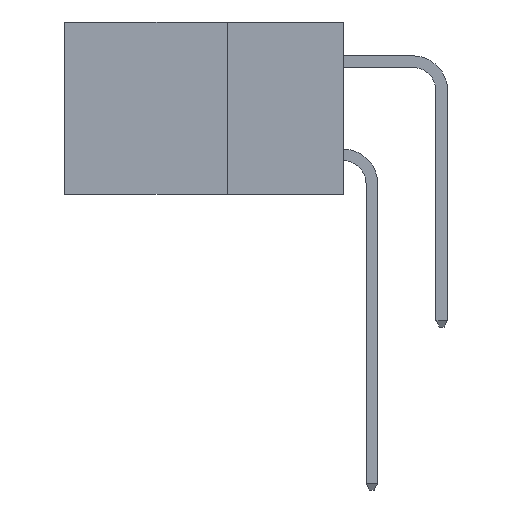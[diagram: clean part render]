
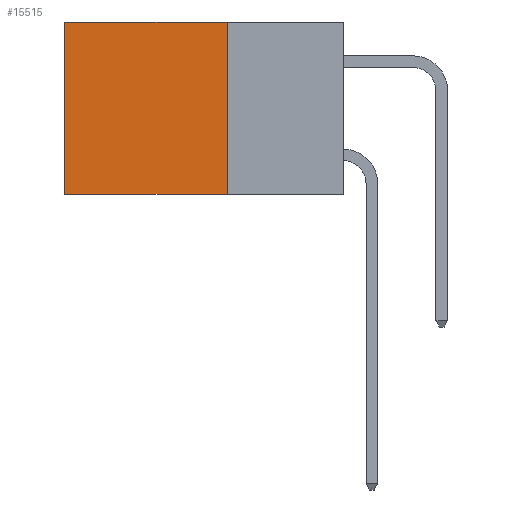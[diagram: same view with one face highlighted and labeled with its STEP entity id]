
A CAD part, left-side view. The second image highlights one B-rep face of the part: STEP entity #15515.
In plain terms, the highlighted planar face has unit normal (-1, 0, 0).
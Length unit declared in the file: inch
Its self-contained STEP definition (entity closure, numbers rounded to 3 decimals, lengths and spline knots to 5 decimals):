
#250 = ORIENTED_EDGE ( 'NONE', *, *, #4271, .F. ) ;
#1023 = FACE_OUTER_BOUND ( 'NONE', #12965, .T. ) ;
#1714 = LINE ( 'NONE', #11186, #11047 ) ;
#1760 = CARTESIAN_POINT ( 'NONE',  ( 0.2615, 0.25, -0.37 ) ) ;
#1818 = DIRECTION ( 'NONE',  ( 0., 1., 0. ) ) ;
#1838 = CARTESIAN_POINT ( 'NONE',  ( 0.2615, 0.25, -0.37 ) ) ;
#2132 = DIRECTION ( 'NONE',  ( 0., 0., -1. ) ) ;
#2157 = CARTESIAN_POINT ( 'NONE',  ( 0.2615, 0.25, 0. ) ) ;
#2179 = DIRECTION ( 'NONE',  ( 1., 0., 0. ) ) ;
#2258 = DIRECTION ( 'NONE',  ( 0., 1., 0. ) ) ;
#2661 = DIRECTION ( 'NONE',  ( 0., 0., -1. ) ) ;
#4271 = EDGE_CURVE ( 'NONE', #15142, #9403, #8372, .T. ) ;
#4823 = VECTOR ( 'NONE', #2258, 39.37008 ) ;
#4864 = CARTESIAN_POINT ( 'NONE',  ( 0.2615, 0.6, -0.37 ) ) ;
#5030 = EDGE_CURVE ( 'NONE', #6784, #15142, #6230, .T. ) ;
#6190 = CARTESIAN_POINT ( 'NONE',  ( 0.2615, 0.25, -0.37 ) ) ;
#6230 = LINE ( 'NONE', #1760, #12434 ) ;
#6784 = VERTEX_POINT ( 'NONE', #9208 ) ;
#8066 = ORIENTED_EDGE ( 'NONE', *, *, #14454, .T. ) ;
#8120 = PLANE ( 'NONE',  #15577 ) ;
#8123 = ORIENTED_EDGE ( 'NONE', *, *, #5030, .F. ) ;
#8372 = LINE ( 'NONE', #1838, #13414 ) ;
#9208 = CARTESIAN_POINT ( 'NONE',  ( 0.2615, 0.25, 0. ) ) ;
#9403 = VERTEX_POINT ( 'NONE', #4864 ) ;
#9445 = CARTESIAN_POINT ( 'NONE',  ( 0.2615, 0.25, -0.37 ) ) ;
#10680 = DIRECTION ( 'NONE',  ( 0., 0., -1. ) ) ;
#10702 = VERTEX_POINT ( 'NONE', #13554 ) ;
#11047 = VECTOR ( 'NONE', #2661, 39.37008 ) ;
#11186 = CARTESIAN_POINT ( 'NONE',  ( 0.2615, 0.6, -0.37 ) ) ;
#12434 = VECTOR ( 'NONE', #2132, 39.37008 ) ;
#12538 = ORIENTED_EDGE ( 'NONE', *, *, #12686, .T. ) ;
#12686 = EDGE_CURVE ( 'NONE', #10702, #9403, #1714, .T. ) ;
#12965 = EDGE_LOOP ( 'NONE', ( #12538, #250, #8123, #8066 ) ) ;
#13414 = VECTOR ( 'NONE', #1818, 39.37008 ) ;
#13554 = CARTESIAN_POINT ( 'NONE',  ( 0.2615, 0.6, 0. ) ) ;
#14454 = EDGE_CURVE ( 'NONE', #6784, #10702, #14903, .T. ) ;
#14903 = LINE ( 'NONE', #2157, #4823 ) ;
#15142 = VERTEX_POINT ( 'NONE', #6190 ) ;
#15515 = ADVANCED_FACE ( 'NONE', ( #1023 ), #8120, .F. ) ;
#15577 = AXIS2_PLACEMENT_3D ( 'NONE', #9445, #2179, #10680 ) ;
